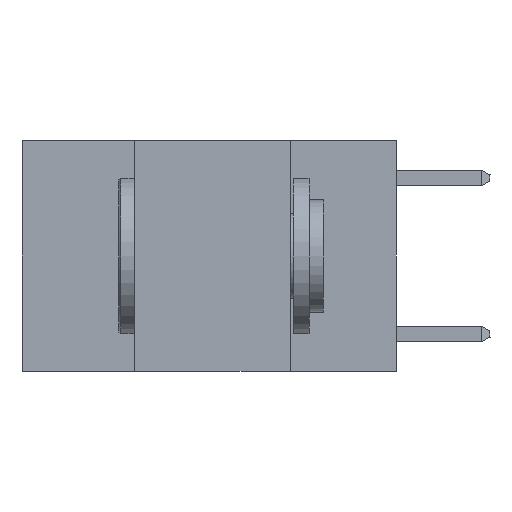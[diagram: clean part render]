
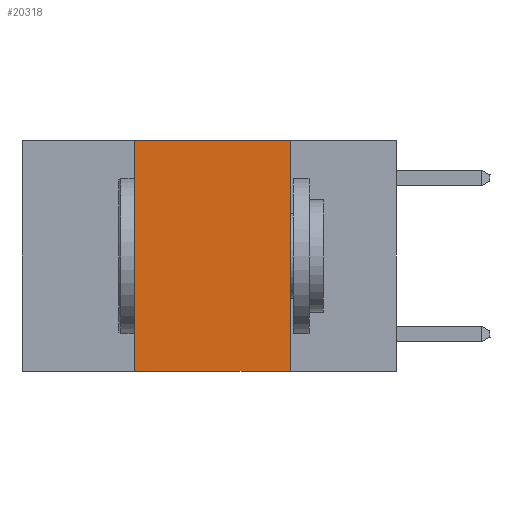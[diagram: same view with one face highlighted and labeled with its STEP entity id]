
A CAD part, left-side view. The second image highlights one B-rep face of the part: STEP entity #20318.
In plain terms, the highlighted planar face has unit normal (-1, 0, 0).
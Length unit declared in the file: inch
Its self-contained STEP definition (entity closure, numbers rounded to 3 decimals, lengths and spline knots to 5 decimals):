
#582 = DIRECTION ( 'NONE',  ( 0., -1., 0. ) ) ;
#936 = DIRECTION ( 'NONE',  ( 0., 0., -1. ) ) ;
#1120 = VERTEX_POINT ( 'NONE', #13524 ) ;
#1638 = VERTEX_POINT ( 'NONE', #7122 ) ;
#1733 = EDGE_CURVE ( 'NONE', #10767, #3689, #9688, .T. ) ;
#1906 = ORIENTED_EDGE ( 'NONE', *, *, #1733, .F. ) ;
#3315 = VECTOR ( 'NONE', #14260, 39.37008 ) ;
#3547 = EDGE_CURVE ( 'NONE', #1638, #10767, #6448, .T. ) ;
#3689 = VERTEX_POINT ( 'NONE', #16394 ) ;
#4401 = DIRECTION ( 'NONE',  ( 1., 0., 0. ) ) ;
#4955 = ORIENTED_EDGE ( 'NONE', *, *, #3547, .F. ) ;
#5862 = FACE_OUTER_BOUND ( 'NONE', #10745, .T. ) ;
#6448 = LINE ( 'NONE', #6941, #13760 ) ;
#6667 = VECTOR ( 'NONE', #582, 39.37008 ) ;
#6780 = EDGE_CURVE ( 'NONE', #3689, #1120, #14040, .T. ) ;
#6941 = CARTESIAN_POINT ( 'NONE',  ( 0., 0.42, 0. ) ) ;
#7122 = CARTESIAN_POINT ( 'NONE',  ( 0., 0.42, -0.37 ) ) ;
#7257 = ORIENTED_EDGE ( 'NONE', *, *, #6780, .F. ) ;
#7448 = PLANE ( 'NONE',  #9571 ) ;
#8090 = ORIENTED_EDGE ( 'NONE', *, *, #8433, .T. ) ;
#8433 = EDGE_CURVE ( 'NONE', #1638, #1120, #11773, .T. ) ;
#9075 = VECTOR ( 'NONE', #19227, 39.37008 ) ;
#9571 = AXIS2_PLACEMENT_3D ( 'NONE', #17009, #4401, #936 ) ;
#9588 = CARTESIAN_POINT ( 'NONE',  ( 0., 0.6, 0. ) ) ;
#9688 = LINE ( 'NONE', #9588, #9075 ) ;
#10745 = EDGE_LOOP ( 'NONE', ( #7257, #1906, #4955, #8090 ) ) ;
#10767 = VERTEX_POINT ( 'NONE', #16725 ) ;
#11773 = LINE ( 'NONE', #16660, #6667 ) ;
#13524 = CARTESIAN_POINT ( 'NONE',  ( 0., 0.17, -0.37 ) ) ;
#13760 = VECTOR ( 'NONE', #19374, 39.37008 ) ;
#14040 = LINE ( 'NONE', #20737, #3315 ) ;
#14260 = DIRECTION ( 'NONE',  ( 0., 0., -1. ) ) ;
#16394 = CARTESIAN_POINT ( 'NONE',  ( 0., 0.17, 0. ) ) ;
#16660 = CARTESIAN_POINT ( 'NONE',  ( 0., 0.6, -0.37 ) ) ;
#16725 = CARTESIAN_POINT ( 'NONE',  ( 0., 0.42, 0. ) ) ;
#17009 = CARTESIAN_POINT ( 'NONE',  ( 0., 0.6, 0. ) ) ;
#19227 = DIRECTION ( 'NONE',  ( 0., -1., 0. ) ) ;
#19374 = DIRECTION ( 'NONE',  ( 0., 0., 1. ) ) ;
#20318 = ADVANCED_FACE ( 'NONE', ( #5862 ), #7448, .F. ) ;
#20737 = CARTESIAN_POINT ( 'NONE',  ( 0., 0.17, 0. ) ) ;
